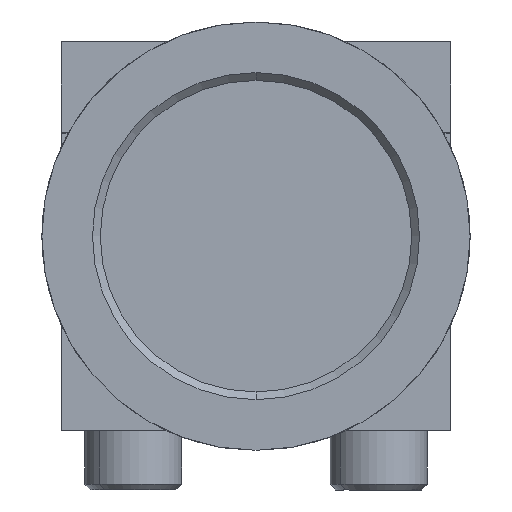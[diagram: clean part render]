
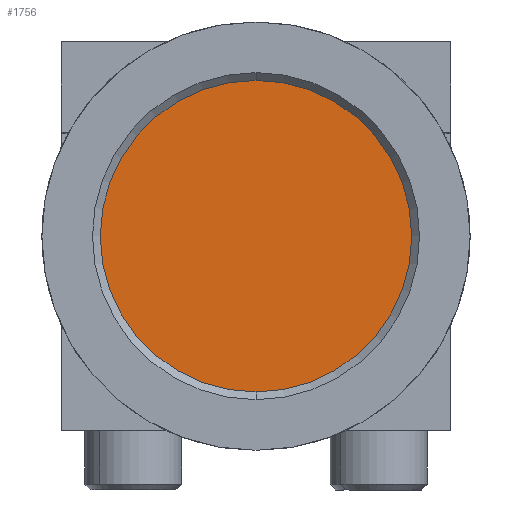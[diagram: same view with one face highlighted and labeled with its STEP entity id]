
A CAD part, front view. The second image highlights one B-rep face of the part: STEP entity #1756.
In plain terms, the highlighted planar face has unit normal (0, -1, 0).
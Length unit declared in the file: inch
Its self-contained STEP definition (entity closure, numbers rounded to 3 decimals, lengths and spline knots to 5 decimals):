
#25 = AXIS2_PLACEMENT_3D ( 'NONE', #1306, #2362, #778 ) ;
#357 = DIRECTION ( 'NONE',  ( 0., 1., 0. ) ) ;
#404 = DIRECTION ( 'NONE',  ( 0., 1., 0. ) ) ;
#778 = DIRECTION ( 'NONE',  ( 0., 0., -1. ) ) ;
#830 = EDGE_CURVE ( 'NONE', #2291, #2152, #2534, .T. ) ;
#973 = AXIS2_PLACEMENT_3D ( 'NONE', #1939, #357, #2195 ) ;
#1129 = CIRCLE ( 'NONE', #973, 0.5 ) ;
#1306 = CARTESIAN_POINT ( 'NONE',  ( 0.625, -0.5, 0. ) ) ;
#1543 = EDGE_CURVE ( 'NONE', #2152, #2291, #1129, .T. ) ;
#1578 = EDGE_LOOP ( 'NONE', ( #2327, #2330 ) ) ;
#1756 = ADVANCED_FACE ( 'NONE', ( #3290 ), #2100, .T. ) ;
#1939 = CARTESIAN_POINT ( 'NONE',  ( 0.625, -0.5, 0. ) ) ;
#1975 = CARTESIAN_POINT ( 'NONE',  ( 0.625, -0.5, 0. ) ) ;
#2023 = CARTESIAN_POINT ( 'NONE',  ( 0.625, -0.5, -0.5 ) ) ;
#2100 = PLANE ( 'NONE',  #25 ) ;
#2118 = AXIS2_PLACEMENT_3D ( 'NONE', #1975, #404, #2244 ) ;
#2152 = VERTEX_POINT ( 'NONE', #2023 ) ;
#2195 = DIRECTION ( 'NONE',  ( 0., 0., 1. ) ) ;
#2244 = DIRECTION ( 'NONE',  ( 0., 0., 1. ) ) ;
#2291 = VERTEX_POINT ( 'NONE', #2865 ) ;
#2327 = ORIENTED_EDGE ( 'NONE', *, *, #830, .F. ) ;
#2330 = ORIENTED_EDGE ( 'NONE', *, *, #1543, .F. ) ;
#2362 = DIRECTION ( 'NONE',  ( 0., -1., 0. ) ) ;
#2534 = CIRCLE ( 'NONE', #2118, 0.5 ) ;
#2865 = CARTESIAN_POINT ( 'NONE',  ( 0.625, -0.5, 0.5 ) ) ;
#3290 = FACE_OUTER_BOUND ( 'NONE', #1578, .T. ) ;
